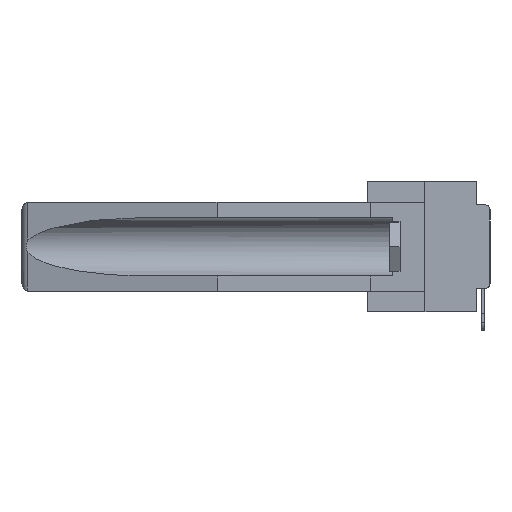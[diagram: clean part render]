
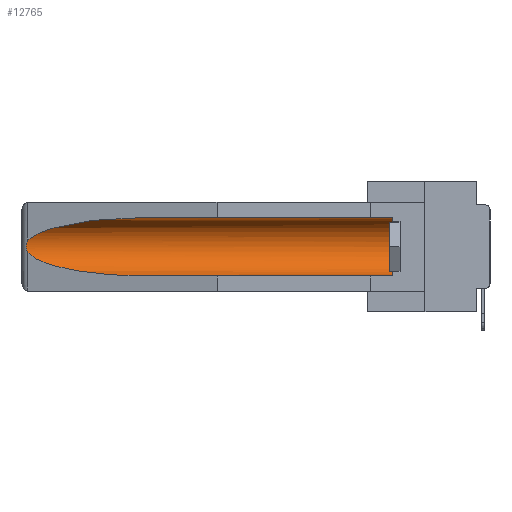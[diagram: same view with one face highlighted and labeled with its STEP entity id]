
A CAD part, left-side view. The second image highlights one B-rep face of the part: STEP entity #12765.
In plain terms, the highlighted cylindrical face has radius 2.857 mm (diameter 5.715 mm), a partial arc.
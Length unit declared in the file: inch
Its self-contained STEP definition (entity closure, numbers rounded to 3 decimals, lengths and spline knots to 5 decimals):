
#165 = ORIENTED_EDGE ( 'NONE', *, *, #26013, .F. ) ;
#619 = CARTESIAN_POINT ( 'NONE',  ( 0.2675, 1.53308, -0.17534 ) ) ;
#627 = CARTESIAN_POINT ( 'NONE',  ( 0.25451, 1.48313, -0.09465 ) ) ;
#737 = CARTESIAN_POINT ( 'NONE',  ( 0.26537, 1.52718, -0.19328 ) ) ;
#1429 = CARTESIAN_POINT ( 'NONE',  ( 0.21114, 1.30732, -0.284 ) ) ;
#1492 = DIRECTION ( 'NONE',  ( 0., 0., 1. ) ) ;
#2694 = DIRECTION ( 'NONE',  ( 0., -1., 0. ) ) ;
#2966 = CARTESIAN_POINT ( 'NONE',  ( 0.26655, 1.53094, -0.18657 ) ) ;
#3108 = CARTESIAN_POINT ( 'NONE',  ( 0.155, 0.126, -0.1715 ) ) ;
#3167 = CARTESIAN_POINT ( 'NONE',  ( 0.26537, 1.52718, -0.14972 ) ) ;
#3689 = CARTESIAN_POINT ( 'NONE',  ( 0.25451, 1.48313, -0.24835 ) ) ;
#5242 = ORIENTED_EDGE ( 'NONE', *, *, #19188, .T. ) ;
#5938 = CARTESIAN_POINT ( 'NONE',  ( 0.155, -0.30754, -0.059 ) ) ;
#6495 = CIRCLE ( 'NONE', #16906, 0.1125 ) ;
#6620 = ORIENTED_EDGE ( 'NONE', *, *, #17625, .T. ) ;
#6699 = CARTESIAN_POINT ( 'NONE',  ( 0.26597, 1.5296, -0.19026 ) ) ;
#6799 = LINE ( 'NONE', #5938, #8633 ) ;
#8633 = VECTOR ( 'NONE', #15199, 39.37008 ) ;
#8858 = EDGE_CURVE ( 'NONE', #17346, #14040, #19303, .T. ) ;
#10339 = CARTESIAN_POINT ( 'NONE',  ( 0.26597, 1.52961, -0.15275 ) ) ;
#11465 = AXIS2_PLACEMENT_3D ( 'NONE', #22509, #17637, #1492 ) ;
#12498 = VERTEX_POINT ( 'NONE', #15863 ) ;
#12609 = CARTESIAN_POINT ( 'NONE',  ( 0.155, 1.07973, -0.059 ) ) ;
#12633 = CARTESIAN_POINT ( 'NONE',  ( 0.2673, 1.5327, -0.16383 ) ) ;
#12765 = ADVANCED_FACE ( 'NONE', ( #24530 ), #20909, .F. ) ;
#13042 = ORIENTED_EDGE ( 'NONE', *, *, #24005, .T. ) ;
#13216 = LINE ( 'NONE', #22601, #23712 ) ;
#13283 = DIRECTION ( 'NONE',  ( 0., 1., 0. ) ) ;
#14022 = EDGE_CURVE ( 'NONE', #28953, #17346, #6799, .T. ) ;
#14040 = VERTEX_POINT ( 'NONE', #15092 ) ;
#14416 = CARTESIAN_POINT ( 'NONE',  ( 0.2675, 1.53308, -0.16763 ) ) ;
#14420 = CARTESIAN_POINT ( 'NONE',  ( 0.21114, 1.30732, -0.059 ) ) ;
#14834 = VERTEX_POINT ( 'NONE', #737 ) ;
#15092 = CARTESIAN_POINT ( 'NONE',  ( 0.26537, 1.52718, -0.14972 ) ) ;
#15126 = CARTESIAN_POINT ( 'NONE',  ( 0.26537, 1.52718, -0.19328 ) ) ;
#15199 = DIRECTION ( 'NONE',  ( 0., 1., 0. ) ) ;
#15530 = CARTESIAN_POINT ( 'NONE',  ( 0.155, 0.126, -0.059 ) ) ;
#15863 = CARTESIAN_POINT ( 'NONE',  ( 0.155, 0.126, -0.284 ) ) ;
#16429 = ORIENTED_EDGE ( 'NONE', *, *, #8858, .T. ) ;
#16759 = CARTESIAN_POINT ( 'NONE',  ( 0.2673, 1.53269, -0.17917 ) ) ;
#16906 = AXIS2_PLACEMENT_3D ( 'NONE', #3108, #2694, #19043 ) ;
#17346 = VERTEX_POINT ( 'NONE', #12609 ) ;
#17625 = EDGE_CURVE ( 'NONE', #12498, #28953, #6495, .T. ) ;
#17637 = DIRECTION ( 'NONE',  ( 0., 1., 0. ) ) ;
#19043 = DIRECTION ( 'NONE',  ( 0., 0., 1. ) ) ;
#19188 = EDGE_CURVE ( 'NONE', #14040, #14834, #22468, .T. ) ;
#19303 =( BOUNDED_CURVE ( )  B_SPLINE_CURVE ( 3, ( #19317, #14420, #627, #21423 ),
 .UNSPECIFIED., .F., .F. ) 
 B_SPLINE_CURVE_WITH_KNOTS ( ( 4, 4 ),
 ( 4.71239, 6.08839 ),
 .UNSPECIFIED. ) 
 CURVE ( )  GEOMETRIC_REPRESENTATION_ITEM ( )  RATIONAL_B_SPLINE_CURVE ( ( 1., 0.848, 0.848, 1. ) ) 
 REPRESENTATION_ITEM ( '' )  );
#19317 = CARTESIAN_POINT ( 'NONE',  ( 0.155, 1.07973, -0.059 ) ) ;
#19730 = ORIENTED_EDGE ( 'NONE', *, *, #14022, .T. ) ;
#20909 = CYLINDRICAL_SURFACE ( 'NONE', #11465, 0.1125 ) ;
#21423 = CARTESIAN_POINT ( 'NONE',  ( 0.26537, 1.52718, -0.14972 ) ) ;
#22468 = B_SPLINE_CURVE_WITH_KNOTS ( 'NONE', 3,
 ( #3167, #10339, #26457, #12633, #14416, #619, #16759, #2966, #6699, #25656 ),
 .UNSPECIFIED., .F., .F.,
 ( 4, 2, 2, 2, 4 ),
 ( 0., 0.00029, 0.00058, 0.00087, 0.00117 ),
 .UNSPECIFIED. ) ;
#22509 = CARTESIAN_POINT ( 'NONE',  ( 0.155, -0.30754, -0.1715 ) ) ;
#22601 = CARTESIAN_POINT ( 'NONE',  ( 0.155, -0.30754, -0.284 ) ) ;
#23712 = VECTOR ( 'NONE', #13283, 39.37008 ) ;
#24005 = EDGE_CURVE ( 'NONE', #14834, #29731, #28298, .T. ) ;
#24530 = FACE_OUTER_BOUND ( 'NONE', #28906, .T. ) ;
#25656 = CARTESIAN_POINT ( 'NONE',  ( 0.26537, 1.52718, -0.19328 ) ) ;
#26013 = EDGE_CURVE ( 'NONE', #12498, #29731, #13216, .T. ) ;
#26451 = CARTESIAN_POINT ( 'NONE',  ( 0.155, 1.07973, -0.284 ) ) ;
#26457 = CARTESIAN_POINT ( 'NONE',  ( 0.26654, 1.53092, -0.15636 ) ) ;
#27858 = CARTESIAN_POINT ( 'NONE',  ( 0.155, 1.07973, -0.284 ) ) ;
#28298 =( BOUNDED_CURVE ( )  B_SPLINE_CURVE ( 3, ( #15126, #3689, #1429, #26451 ),
 .UNSPECIFIED., .F., .F. ) 
 B_SPLINE_CURVE_WITH_KNOTS ( ( 4, 4 ),
 ( 0.1948, 1.5708 ),
 .UNSPECIFIED. ) 
 CURVE ( )  GEOMETRIC_REPRESENTATION_ITEM ( )  RATIONAL_B_SPLINE_CURVE ( ( 1., 0.848, 0.848, 1. ) ) 
 REPRESENTATION_ITEM ( '' )  );
#28906 = EDGE_LOOP ( 'NONE', ( #16429, #5242, #13042, #165, #6620, #19730 ) ) ;
#28953 = VERTEX_POINT ( 'NONE', #15530 ) ;
#29731 = VERTEX_POINT ( 'NONE', #27858 ) ;
